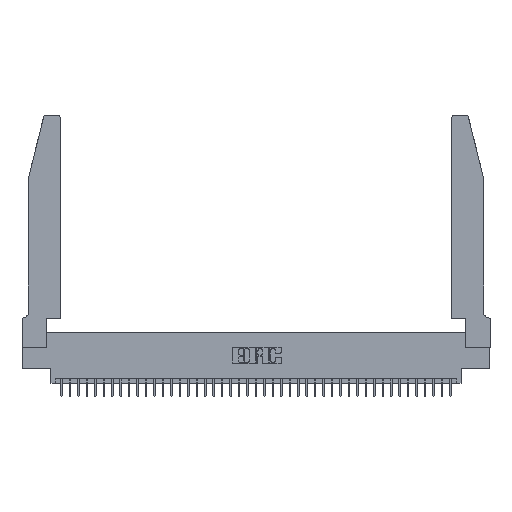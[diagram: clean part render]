
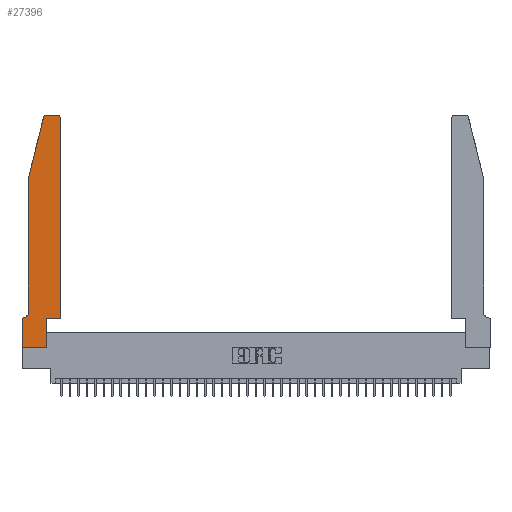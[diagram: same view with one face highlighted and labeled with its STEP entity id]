
A CAD part, top view. The second image highlights one B-rep face of the part: STEP entity #27396.
In plain terms, the highlighted planar face has unit normal (0, 0, 1).
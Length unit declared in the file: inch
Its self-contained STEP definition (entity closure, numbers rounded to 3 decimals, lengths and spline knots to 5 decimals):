
#1301 = CARTESIAN_POINT ( 'NONE',  ( 0.0755, 2., 0.37 ) ) ;
#1968 = VECTOR ( 'NONE', #4575, 39.37008 ) ;
#2617 = EDGE_CURVE ( 'NONE', #10361, #24172, #17603, .T. ) ;
#2769 = CARTESIAN_POINT ( 'NONE',  ( 0., 0., 0.37 ) ) ;
#2981 = LINE ( 'NONE', #1301, #1968 ) ;
#3301 = EDGE_CURVE ( 'NONE', #11679, #8887, #17036, .T. ) ;
#3793 = CARTESIAN_POINT ( 'NONE',  ( 0.4205, 2.75, 0.37 ) ) ;
#3964 = DIRECTION ( 'NONE',  ( 0., 1., 0. ) ) ;
#4082 = ORIENTED_EDGE ( 'NONE', *, *, #34300, .T. ) ;
#4575 = DIRECTION ( 'NONE',  ( -0.239, -0.971, 0. ) ) ;
#4577 = DIRECTION ( 'NONE',  ( 1., 0., 0. ) ) ;
#4620 = DIRECTION ( 'NONE',  ( 0., 0., 1. ) ) ;
#4745 = ORIENTED_EDGE ( 'NONE', *, *, #13782, .T. ) ;
#5476 = CARTESIAN_POINT ( 'NONE',  ( 0.0755, 2., 0.37 ) ) ;
#6042 = EDGE_CURVE ( 'NONE', #35671, #20629, #11871, .T. ) ;
#6531 = CARTESIAN_POINT ( 'NONE',  ( 0.2865, 0., 0.37 ) ) ;
#7466 = VERTEX_POINT ( 'NONE', #28865 ) ;
#7543 = ORIENTED_EDGE ( 'NONE', *, *, #16183, .T. ) ;
#7752 = AXIS2_PLACEMENT_3D ( 'NONE', #18655, #40646, #21824 ) ;
#7874 = VECTOR ( 'NONE', #38825, 39.37008 ) ;
#8317 = AXIS2_PLACEMENT_3D ( 'NONE', #12367, #9243, #31470 ) ;
#8887 = VERTEX_POINT ( 'NONE', #15438 ) ;
#9243 = DIRECTION ( 'NONE',  ( 0., 0., 1. ) ) ;
#9494 = VECTOR ( 'NONE', #35161, 39.37008 ) ;
#9507 = VERTEX_POINT ( 'NONE', #24392 ) ;
#9839 = CARTESIAN_POINT ( 'NONE',  ( 0.0755, 2., 0.37 ) ) ;
#10106 = EDGE_CURVE ( 'NONE', #30922, #35671, #38931, .T. ) ;
#10361 = VERTEX_POINT ( 'NONE', #15475 ) ;
#10696 = ORIENTED_EDGE ( 'NONE', *, *, #6042, .T. ) ;
#11679 = VERTEX_POINT ( 'NONE', #5476 ) ;
#11871 = LINE ( 'NONE', #15557, #37078 ) ;
#12125 = VERTEX_POINT ( 'NONE', #14969 ) ;
#12367 = CARTESIAN_POINT ( 'NONE',  ( 0., 0.35, 0.37 ) ) ;
#12567 = CARTESIAN_POINT ( 'NONE',  ( 0., 0.35, 0.37 ) ) ;
#12653 = CARTESIAN_POINT ( 'NONE',  ( 0.25487, 2.72718, 0.37 ) ) ;
#12748 = VECTOR ( 'NONE', #4577, 39.37008 ) ;
#12944 = CARTESIAN_POINT ( 'NONE',  ( 0.0055, 0.42, 0.37 ) ) ;
#13376 = EDGE_LOOP ( 'NONE', ( #7543, #38458, #4082, #36602, #38429, #19254, #21061, #41145, #10696, #4745, #19469, #18491 ) ) ;
#13782 = EDGE_CURVE ( 'NONE', #20629, #9507, #40571, .T. ) ;
#14220 = CARTESIAN_POINT ( 'NONE',  ( 0., 0., 0.37 ) ) ;
#14969 = CARTESIAN_POINT ( 'NONE',  ( 0.284, 2.75, 0.37 ) ) ;
#15438 = CARTESIAN_POINT ( 'NONE',  ( 0.0755, 0.42, 0.37 ) ) ;
#15475 = CARTESIAN_POINT ( 'NONE',  ( 0.4505, 2.72, 0.37 ) ) ;
#15557 = CARTESIAN_POINT ( 'NONE',  ( 0.2865, 0.35, 0.37 ) ) ;
#15575 = LINE ( 'NONE', #36555, #16996 ) ;
#15749 = CARTESIAN_POINT ( 'NONE',  ( 0.2865, 0.35, 0.37 ) ) ;
#16174 = DIRECTION ( 'NONE',  ( -1., 0., 0. ) ) ;
#16183 = EDGE_CURVE ( 'NONE', #24172, #12125, #26147, .T. ) ;
#16996 = VECTOR ( 'NONE', #17723, 39.37008 ) ;
#17036 = LINE ( 'NONE', #9839, #9494 ) ;
#17603 = CIRCLE ( 'NONE', #7752, 0.03 ) ;
#17723 = DIRECTION ( 'NONE',  ( 0., -1., 0. ) ) ;
#17993 = CIRCLE ( 'NONE', #34205, 0.07 ) ;
#18491 = ORIENTED_EDGE ( 'NONE', *, *, #2617, .T. ) ;
#18655 = CARTESIAN_POINT ( 'NONE',  ( 0.4205, 2.72, 0.37 ) ) ;
#19254 = ORIENTED_EDGE ( 'NONE', *, *, #39287, .T. ) ;
#19377 = DIRECTION ( 'NONE',  ( -1., 0., 0. ) ) ;
#19469 = ORIENTED_EDGE ( 'NONE', *, *, #27653, .T. ) ;
#19981 = CARTESIAN_POINT ( 'NONE',  ( 0.4505, 0.35, 0.37 ) ) ;
#20022 = CARTESIAN_POINT ( 'NONE',  ( 0.4505, 0.35, 0.37 ) ) ;
#20048 = AXIS2_PLACEMENT_3D ( 'NONE', #23840, #4620, #26998 ) ;
#20629 = VERTEX_POINT ( 'NONE', #15749 ) ;
#21061 = ORIENTED_EDGE ( 'NONE', *, *, #31316, .T. ) ;
#21824 = DIRECTION ( 'NONE',  ( 1., 0., 0. ) ) ;
#23468 = EDGE_CURVE ( 'NONE', #12125, #29400, #33615, .T. ) ;
#23840 = CARTESIAN_POINT ( 'NONE',  ( 0.284, 2.72, 0.37 ) ) ;
#24172 = VERTEX_POINT ( 'NONE', #3793 ) ;
#24392 = CARTESIAN_POINT ( 'NONE',  ( 0.4505, 0.35, 0.37 ) ) ;
#24673 = VERTEX_POINT ( 'NONE', #12567 ) ;
#25618 = CARTESIAN_POINT ( 'NONE',  ( 0.0755, 0.35, 0.37 ) ) ;
#25733 = VECTOR ( 'NONE', #3964, 39.37008 ) ;
#26147 = LINE ( 'NONE', #32363, #34502 ) ;
#26224 = FACE_OUTER_BOUND ( 'NONE', #13376, .T. ) ;
#26998 = DIRECTION ( 'NONE',  ( 1., 0., 0. ) ) ;
#27396 = ADVANCED_FACE ( 'NONE', ( #26224 ), #28315, .T. ) ;
#27653 = EDGE_CURVE ( 'NONE', #9507, #10361, #34074, .T. ) ;
#28315 = PLANE ( 'NONE',  #8317 ) ;
#28865 = CARTESIAN_POINT ( 'NONE',  ( 0.0055, 0.35, 0.37 ) ) ;
#29400 = VERTEX_POINT ( 'NONE', #12653 ) ;
#30627 = VECTOR ( 'NONE', #19377, 39.37008 ) ;
#30922 = VERTEX_POINT ( 'NONE', #2769 ) ;
#31316 = EDGE_CURVE ( 'NONE', #24673, #30922, #15575, .T. ) ;
#31470 = DIRECTION ( 'NONE',  ( 1., 0., 0. ) ) ;
#32363 = CARTESIAN_POINT ( 'NONE',  ( 0.2605, 2.75, 0.37 ) ) ;
#33615 = CIRCLE ( 'NONE', #20048, 0.03 ) ;
#34074 = LINE ( 'NONE', #20022, #25733 ) ;
#34205 = AXIS2_PLACEMENT_3D ( 'NONE', #12944, #35034, #16174 ) ;
#34300 = EDGE_CURVE ( 'NONE', #29400, #11679, #2981, .T. ) ;
#34431 = DIRECTION ( 'NONE',  ( 0., 1., 0. ) ) ;
#34502 = VECTOR ( 'NONE', #35492, 39.37008 ) ;
#35034 = DIRECTION ( 'NONE',  ( 0., 0., -1. ) ) ;
#35161 = DIRECTION ( 'NONE',  ( 0., -1., 0. ) ) ;
#35492 = DIRECTION ( 'NONE',  ( -1., 0., 0. ) ) ;
#35671 = VERTEX_POINT ( 'NONE', #6531 ) ;
#36555 = CARTESIAN_POINT ( 'NONE',  ( 0., 0., 0.37 ) ) ;
#36602 = ORIENTED_EDGE ( 'NONE', *, *, #3301, .T. ) ;
#36947 = EDGE_CURVE ( 'NONE', #8887, #7466, #17993, .T. ) ;
#37078 = VECTOR ( 'NONE', #34431, 39.37008 ) ;
#38429 = ORIENTED_EDGE ( 'NONE', *, *, #36947, .T. ) ;
#38458 = ORIENTED_EDGE ( 'NONE', *, *, #23468, .T. ) ;
#38825 = DIRECTION ( 'NONE',  ( 1., 0., 0. ) ) ;
#38931 = LINE ( 'NONE', #14220, #12748 ) ;
#38958 = LINE ( 'NONE', #25618, #30627 ) ;
#39287 = EDGE_CURVE ( 'NONE', #7466, #24673, #38958, .T. ) ;
#40571 = LINE ( 'NONE', #19981, #7874 ) ;
#40646 = DIRECTION ( 'NONE',  ( 0., 0., 1. ) ) ;
#41145 = ORIENTED_EDGE ( 'NONE', *, *, #10106, .T. ) ;
